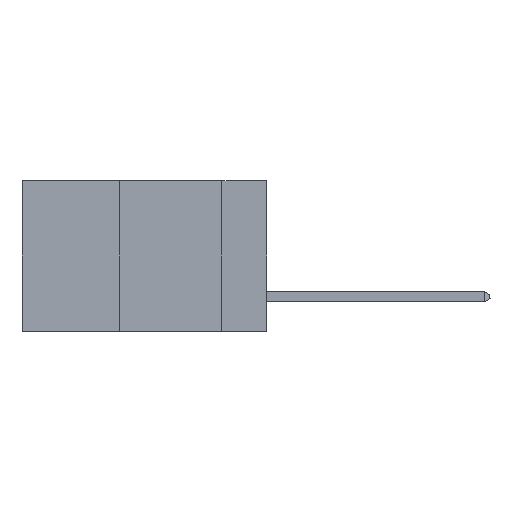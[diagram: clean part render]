
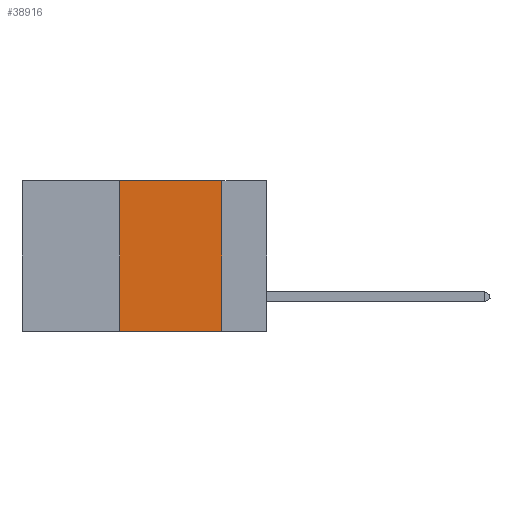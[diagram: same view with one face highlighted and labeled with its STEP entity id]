
A CAD part, left-side view. The second image highlights one B-rep face of the part: STEP entity #38916.
In plain terms, the highlighted planar face has unit normal (-1, 0, 0).
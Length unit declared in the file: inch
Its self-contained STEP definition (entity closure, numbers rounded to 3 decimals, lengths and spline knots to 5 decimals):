
#619 = LINE ( 'NONE', #23872, #2646 ) ;
#1556 = VERTEX_POINT ( 'NONE', #29423 ) ;
#2646 = VECTOR ( 'NONE', #5250, 39.37008 ) ;
#2648 = DIRECTION ( 'NONE',  ( 0., 0., 1. ) ) ;
#5250 = DIRECTION ( 'NONE',  ( 0., -1., 0. ) ) ;
#6671 = ORIENTED_EDGE ( 'NONE', *, *, #12624, .F. ) ;
#8848 = VECTOR ( 'NONE', #2648, 39.37008 ) ;
#12624 = EDGE_CURVE ( 'NONE', #1556, #14821, #34322, .T. ) ;
#14821 = VERTEX_POINT ( 'NONE', #22293 ) ;
#15316 = VERTEX_POINT ( 'NONE', #17490 ) ;
#15432 = CARTESIAN_POINT ( 'NONE',  ( 0., 0.6, 0. ) ) ;
#15867 = EDGE_LOOP ( 'NONE', ( #19391, #6671, #22364, #29994 ) ) ;
#17490 = CARTESIAN_POINT ( 'NONE',  ( 0., 0.11, -0.37 ) ) ;
#18245 = VECTOR ( 'NONE', #27946, 39.37008 ) ;
#18429 = EDGE_CURVE ( 'NONE', #14821, #15316, #23523, .T. ) ;
#19391 = ORIENTED_EDGE ( 'NONE', *, *, #18429, .F. ) ;
#21109 = CARTESIAN_POINT ( 'NONE',  ( 0., 0.36, 0. ) ) ;
#21326 = DIRECTION ( 'NONE',  ( 0., 0., -1. ) ) ;
#22293 = CARTESIAN_POINT ( 'NONE',  ( 0., 0.11, 0. ) ) ;
#22364 = ORIENTED_EDGE ( 'NONE', *, *, #36955, .F. ) ;
#23523 = LINE ( 'NONE', #30784, #18245 ) ;
#23872 = CARTESIAN_POINT ( 'NONE',  ( 0., 0.6, -0.37 ) ) ;
#24293 = LINE ( 'NONE', #21109, #8848 ) ;
#24817 = DIRECTION ( 'NONE',  ( 1., 0., 0. ) ) ;
#26481 = DIRECTION ( 'NONE',  ( 0., -1., 0. ) ) ;
#27211 = EDGE_CURVE ( 'NONE', #33968, #15316, #619, .T. ) ;
#27946 = DIRECTION ( 'NONE',  ( 0., 0., -1. ) ) ;
#29423 = CARTESIAN_POINT ( 'NONE',  ( 0., 0.36, 0. ) ) ;
#29994 = ORIENTED_EDGE ( 'NONE', *, *, #27211, .T. ) ;
#30784 = CARTESIAN_POINT ( 'NONE',  ( 0., 0.11, 0. ) ) ;
#33946 = CARTESIAN_POINT ( 'NONE',  ( 0., 0.36, -0.37 ) ) ;
#33968 = VERTEX_POINT ( 'NONE', #33946 ) ;
#34322 = LINE ( 'NONE', #34500, #36305 ) ;
#34500 = CARTESIAN_POINT ( 'NONE',  ( 0., 0.6, 0. ) ) ;
#36305 = VECTOR ( 'NONE', #26481, 39.37008 ) ;
#36955 = EDGE_CURVE ( 'NONE', #33968, #1556, #24293, .T. ) ;
#36959 = FACE_OUTER_BOUND ( 'NONE', #15867, .T. ) ;
#38193 = AXIS2_PLACEMENT_3D ( 'NONE', #15432, #24817, #21326 ) ;
#38916 = ADVANCED_FACE ( 'NONE', ( #36959 ), #39761, .F. ) ;
#39761 = PLANE ( 'NONE',  #38193 ) ;
